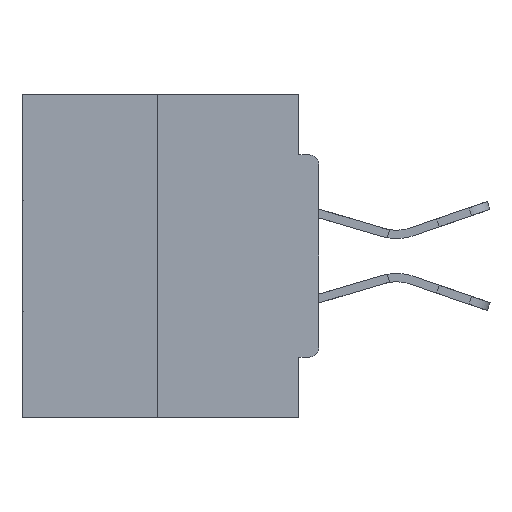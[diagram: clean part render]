
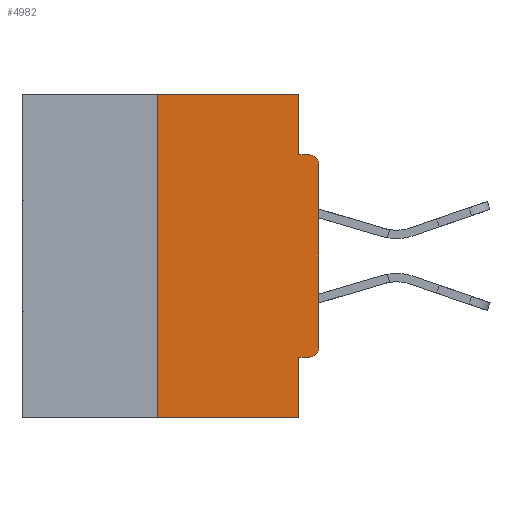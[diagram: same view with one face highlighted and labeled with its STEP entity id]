
A CAD part, left-side view. The second image highlights one B-rep face of the part: STEP entity #4982.
In plain terms, the highlighted planar face has unit normal (-1, 0, 0).
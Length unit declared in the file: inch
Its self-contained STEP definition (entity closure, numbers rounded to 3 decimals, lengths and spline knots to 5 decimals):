
#133 = DIRECTION ( 'NONE',  ( 0., 0., 1. ) ) ;
#578 = VECTOR ( 'NONE', #35386, 39.37008 ) ;
#855 = CARTESIAN_POINT ( 'NONE',  ( 0., 0.25, 0. ) ) ;
#1959 = VERTEX_POINT ( 'NONE', #22723 ) ;
#2269 = EDGE_CURVE ( 'NONE', #1959, #9086, #22258, .T. ) ;
#4004 = CARTESIAN_POINT ( 'NONE',  ( 0., 0.25, -0.5 ) ) ;
#4051 = EDGE_CURVE ( 'NONE', #33777, #29189, #37186, .T. ) ;
#4624 = AXIS2_PLACEMENT_3D ( 'NONE', #28683, #28416, #7075 ) ;
#4841 = CARTESIAN_POINT ( 'NONE',  ( 0., 0.46, -0.5 ) ) ;
#4982 = ADVANCED_FACE ( 'NONE', ( #30406 ), #17451, .F. ) ;
#5849 = LINE ( 'NONE', #32461, #578 ) ;
#5901 = CARTESIAN_POINT ( 'NONE',  ( 0., 0., 0. ) ) ;
#6365 = VECTOR ( 'NONE', #15247, 39.37008 ) ;
#6419 = EDGE_CURVE ( 'NONE', #23428, #1959, #28851, .T. ) ;
#7075 = DIRECTION ( 'NONE',  ( 0., 0., -1. ) ) ;
#7305 = LINE ( 'NONE', #4841, #6365 ) ;
#7941 = VECTOR ( 'NONE', #133, 39.37008 ) ;
#8016 = EDGE_CURVE ( 'NONE', #9086, #33142, #33079, .T. ) ;
#9086 = VERTEX_POINT ( 'NONE', #37336 ) ;
#9420 = ORIENTED_EDGE ( 'NONE', *, *, #12909, .F. ) ;
#9658 = AXIS2_PLACEMENT_3D ( 'NONE', #26103, #29208, #38842 ) ;
#10215 = CARTESIAN_POINT ( 'NONE',  ( 0., 0.031, -0.4065 ) ) ;
#10809 = CARTESIAN_POINT ( 'NONE',  ( 0., 0.015, -0.4065 ) ) ;
#12851 = VECTOR ( 'NONE', #14305, 39.37008 ) ;
#12909 = EDGE_CURVE ( 'NONE', #23428, #19981, #27917, .T. ) ;
#13128 = DIRECTION ( 'NONE',  ( 0., 0., -1. ) ) ;
#13735 = ORIENTED_EDGE ( 'NONE', *, *, #31900, .F. ) ;
#14305 = DIRECTION ( 'NONE',  ( 0., 0., 1. ) ) ;
#15237 = LINE ( 'NONE', #17504, #12851 ) ;
#15247 = DIRECTION ( 'NONE',  ( 0., -1., 0. ) ) ;
#15933 = CARTESIAN_POINT ( 'NONE',  ( 0., 0.031, -0.5 ) ) ;
#16087 = CARTESIAN_POINT ( 'NONE',  ( 0., 0.031, -0.0935 ) ) ;
#16107 = ORIENTED_EDGE ( 'NONE', *, *, #32233, .F. ) ;
#17436 = VECTOR ( 'NONE', #18693, 39.37008 ) ;
#17451 = PLANE ( 'NONE',  #9658 ) ;
#17504 = CARTESIAN_POINT ( 'NONE',  ( 0., 0.25, 0. ) ) ;
#18693 = DIRECTION ( 'NONE',  ( 0., 1., 0. ) ) ;
#18866 = ORIENTED_EDGE ( 'NONE', *, *, #6419, .T. ) ;
#19981 = VERTEX_POINT ( 'NONE', #10215 ) ;
#20083 = ORIENTED_EDGE ( 'NONE', *, *, #37672, .T. ) ;
#20553 = DIRECTION ( 'NONE',  ( 0., 0., -1. ) ) ;
#20627 = EDGE_LOOP ( 'NONE', ( #29844, #27723, #20083, #13735, #9420, #18866, #37939, #37471, #16107, #37214 ) ) ;
#20747 = DIRECTION ( 'NONE',  ( 0., -1., 0. ) ) ;
#20838 = EDGE_CURVE ( 'NONE', #29189, #24050, #5849, .T. ) ;
#22004 = CARTESIAN_POINT ( 'NONE',  ( 0., 0.015, -0.0935 ) ) ;
#22258 = LINE ( 'NONE', #5901, #7941 ) ;
#22311 = LINE ( 'NONE', #15933, #33798 ) ;
#22723 = CARTESIAN_POINT ( 'NONE',  ( 0., 0., -0.3915 ) ) ;
#23428 = VERTEX_POINT ( 'NONE', #10809 ) ;
#24050 = VERTEX_POINT ( 'NONE', #16087 ) ;
#24194 = LINE ( 'NONE', #39194, #32791 ) ;
#26103 = CARTESIAN_POINT ( 'NONE',  ( 0., 0.46, 0. ) ) ;
#27590 = AXIS2_PLACEMENT_3D ( 'NONE', #30162, #38998, #20553 ) ;
#27723 = ORIENTED_EDGE ( 'NONE', *, *, #30421, .F. ) ;
#27917 = LINE ( 'NONE', #33782, #17436 ) ;
#28107 = DIRECTION ( 'NONE',  ( 0., -1., 0. ) ) ;
#28416 = DIRECTION ( 'NONE',  ( -1., 0., 0. ) ) ;
#28683 = CARTESIAN_POINT ( 'NONE',  ( 0., 0.015, -0.1085 ) ) ;
#28851 = CIRCLE ( 'NONE', #27590, 0.015 ) ;
#29189 = VERTEX_POINT ( 'NONE', #39263 ) ;
#29208 = DIRECTION ( 'NONE',  ( 1., 0., 0. ) ) ;
#29559 = VECTOR ( 'NONE', #28107, 39.37008 ) ;
#29844 = ORIENTED_EDGE ( 'NONE', *, *, #4051, .F. ) ;
#30162 = CARTESIAN_POINT ( 'NONE',  ( 0., 0.015, -0.3915 ) ) ;
#30406 = FACE_OUTER_BOUND ( 'NONE', #20627, .T. ) ;
#30421 = EDGE_CURVE ( 'NONE', #34292, #33777, #15237, .T. ) ;
#31188 = CARTESIAN_POINT ( 'NONE',  ( 0., 0.46, 0. ) ) ;
#31222 = VERTEX_POINT ( 'NONE', #33908 ) ;
#31900 = EDGE_CURVE ( 'NONE', #19981, #31222, #22311, .T. ) ;
#32233 = EDGE_CURVE ( 'NONE', #24050, #33142, #24194, .T. ) ;
#32461 = CARTESIAN_POINT ( 'NONE',  ( 0., 0.031, 0. ) ) ;
#32791 = VECTOR ( 'NONE', #20747, 39.37008 ) ;
#33079 = CIRCLE ( 'NONE', #4624, 0.015 ) ;
#33142 = VERTEX_POINT ( 'NONE', #22004 ) ;
#33777 = VERTEX_POINT ( 'NONE', #855 ) ;
#33782 = CARTESIAN_POINT ( 'NONE',  ( 0., 0., -0.4065 ) ) ;
#33798 = VECTOR ( 'NONE', #13128, 39.37008 ) ;
#33908 = CARTESIAN_POINT ( 'NONE',  ( 0., 0.031, -0.5 ) ) ;
#34292 = VERTEX_POINT ( 'NONE', #4004 ) ;
#35386 = DIRECTION ( 'NONE',  ( 0., 0., -1. ) ) ;
#37186 = LINE ( 'NONE', #31188, #29559 ) ;
#37214 = ORIENTED_EDGE ( 'NONE', *, *, #20838, .F. ) ;
#37336 = CARTESIAN_POINT ( 'NONE',  ( 0., 0., -0.1085 ) ) ;
#37471 = ORIENTED_EDGE ( 'NONE', *, *, #8016, .T. ) ;
#37672 = EDGE_CURVE ( 'NONE', #34292, #31222, #7305, .T. ) ;
#37939 = ORIENTED_EDGE ( 'NONE', *, *, #2269, .T. ) ;
#38842 = DIRECTION ( 'NONE',  ( 0., 0., -1. ) ) ;
#38998 = DIRECTION ( 'NONE',  ( -1., 0., 0. ) ) ;
#39194 = CARTESIAN_POINT ( 'NONE',  ( 0., 0., -0.0935 ) ) ;
#39263 = CARTESIAN_POINT ( 'NONE',  ( 0., 0.031, 0. ) ) ;
